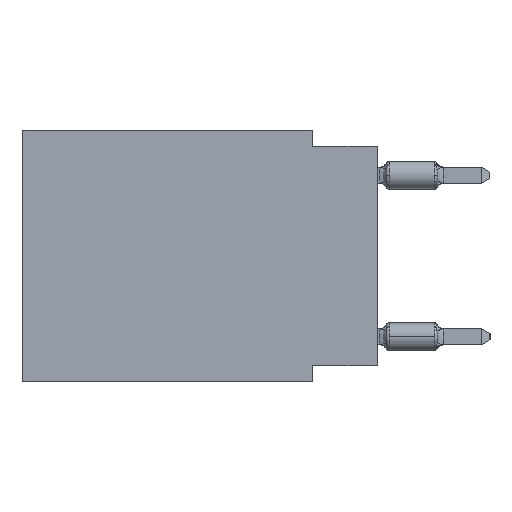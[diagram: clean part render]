
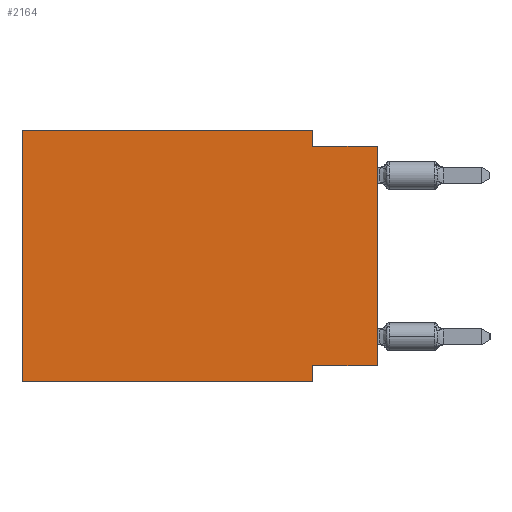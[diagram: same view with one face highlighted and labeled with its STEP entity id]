
A CAD part, left-side view. The second image highlights one B-rep face of the part: STEP entity #2164.
In plain terms, the highlighted planar face has unit normal (-1, 0, 0).
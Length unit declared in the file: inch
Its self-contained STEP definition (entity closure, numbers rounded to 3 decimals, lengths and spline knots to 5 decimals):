
#713 = CARTESIAN_POINT ( 'NONE',  ( 0., 0., 0. ) ) ;
#2164 = ADVANCED_FACE ( 'NONE', ( #4835 ), #30822, .F. ) ;
#2809 = CARTESIAN_POINT ( 'NONE',  ( 0., 0.55, 0. ) ) ;
#2903 = VERTEX_POINT ( 'NONE', #6981 ) ;
#3348 = EDGE_CURVE ( 'NONE', #12321, #16263, #21961, .T. ) ;
#3411 = CARTESIAN_POINT ( 'NONE',  ( 0., 0.1, -0.39 ) ) ;
#3478 = CARTESIAN_POINT ( 'NONE',  ( 0., 0.1, -0.365 ) ) ;
#3516 = VERTEX_POINT ( 'NONE', #37759 ) ;
#4691 = LINE ( 'NONE', #11243, #46310 ) ;
#4835 = FACE_OUTER_BOUND ( 'NONE', #22548, .T. ) ;
#5545 = VECTOR ( 'NONE', #43351, 39.37008 ) ;
#6262 = AXIS2_PLACEMENT_3D ( 'NONE', #34240, #31296, #8716 ) ;
#6981 = CARTESIAN_POINT ( 'NONE',  ( 0., 0., -0.365 ) ) ;
#7005 = CARTESIAN_POINT ( 'NONE',  ( 0., 0.55, -0.39 ) ) ;
#8716 = DIRECTION ( 'NONE',  ( 0., 0., -1. ) ) ;
#8881 = EDGE_CURVE ( 'NONE', #2903, #16263, #44655, .T. ) ;
#9873 = CARTESIAN_POINT ( 'NONE',  ( 0., 0.1, -0.39 ) ) ;
#10056 = ORIENTED_EDGE ( 'NONE', *, *, #18883, .F. ) ;
#10548 = CARTESIAN_POINT ( 'NONE',  ( 0., 0., -0.025 ) ) ;
#10950 = LINE ( 'NONE', #25783, #45664 ) ;
#11243 = CARTESIAN_POINT ( 'NONE',  ( 0., 0.55, 0. ) ) ;
#11287 = EDGE_CURVE ( 'NONE', #3516, #16032, #31505, .T. ) ;
#12321 = VERTEX_POINT ( 'NONE', #26258 ) ;
#12491 = CARTESIAN_POINT ( 'NONE',  ( 0., 0., -0.025 ) ) ;
#13269 = DIRECTION ( 'NONE',  ( 0., 0., 1. ) ) ;
#13389 = ORIENTED_EDGE ( 'NONE', *, *, #41497, .T. ) ;
#16032 = VERTEX_POINT ( 'NONE', #2809 ) ;
#16173 = CARTESIAN_POINT ( 'NONE',  ( 0., 0.1, 0. ) ) ;
#16263 = VERTEX_POINT ( 'NONE', #12491 ) ;
#17025 = VECTOR ( 'NONE', #32814, 39.37008 ) ;
#18883 = EDGE_CURVE ( 'NONE', #31305, #30698, #44447, .T. ) ;
#19387 = EDGE_CURVE ( 'NONE', #47445, #12321, #32511, .T. ) ;
#21961 = LINE ( 'NONE', #10548, #5545 ) ;
#22127 = DIRECTION ( 'NONE',  ( 0., 1., 0. ) ) ;
#22436 = EDGE_CURVE ( 'NONE', #16032, #47445, #4691, .T. ) ;
#22548 = EDGE_LOOP ( 'NONE', ( #25503, #32218, #28110, #30426, #34931, #13389, #10056, #30839 ) ) ;
#23762 = DIRECTION ( 'NONE',  ( 0., 0., 1. ) ) ;
#25210 = DIRECTION ( 'NONE',  ( 0., 0., -1. ) ) ;
#25503 = ORIENTED_EDGE ( 'NONE', *, *, #8881, .T. ) ;
#25783 = CARTESIAN_POINT ( 'NONE',  ( 0., 0., -0.365 ) ) ;
#26258 = CARTESIAN_POINT ( 'NONE',  ( 0., 0.1, -0.025 ) ) ;
#28110 = ORIENTED_EDGE ( 'NONE', *, *, #19387, .F. ) ;
#30206 = DIRECTION ( 'NONE',  ( 0., -1., 0. ) ) ;
#30426 = ORIENTED_EDGE ( 'NONE', *, *, #22436, .F. ) ;
#30698 = VERTEX_POINT ( 'NONE', #9873 ) ;
#30822 = PLANE ( 'NONE',  #6262 ) ;
#30839 = ORIENTED_EDGE ( 'NONE', *, *, #36082, .F. ) ;
#31296 = DIRECTION ( 'NONE',  ( 1., 0., 0. ) ) ;
#31305 = VERTEX_POINT ( 'NONE', #3478 ) ;
#31505 = LINE ( 'NONE', #39271, #31785 ) ;
#31785 = VECTOR ( 'NONE', #13269, 39.37008 ) ;
#32218 = ORIENTED_EDGE ( 'NONE', *, *, #3348, .F. ) ;
#32511 = LINE ( 'NONE', #39550, #44769 ) ;
#32814 = DIRECTION ( 'NONE',  ( 0., 0., -1. ) ) ;
#34240 = CARTESIAN_POINT ( 'NONE',  ( 0., 0.55, 0. ) ) ;
#34931 = ORIENTED_EDGE ( 'NONE', *, *, #11287, .F. ) ;
#36082 = EDGE_CURVE ( 'NONE', #2903, #31305, #10950, .T. ) ;
#37759 = CARTESIAN_POINT ( 'NONE',  ( 0., 0.55, -0.39 ) ) ;
#39271 = CARTESIAN_POINT ( 'NONE',  ( 0., 0.55, 0. ) ) ;
#39313 = VECTOR ( 'NONE', #23762, 39.37008 ) ;
#39550 = CARTESIAN_POINT ( 'NONE',  ( 0., 0.1, 0. ) ) ;
#40265 = LINE ( 'NONE', #7005, #45212 ) ;
#41497 = EDGE_CURVE ( 'NONE', #3516, #30698, #40265, .T. ) ;
#43351 = DIRECTION ( 'NONE',  ( 0., -1., 0. ) ) ;
#44447 = LINE ( 'NONE', #3411, #17025 ) ;
#44655 = LINE ( 'NONE', #713, #39313 ) ;
#44769 = VECTOR ( 'NONE', #25210, 39.37008 ) ;
#45212 = VECTOR ( 'NONE', #47482, 39.37008 ) ;
#45664 = VECTOR ( 'NONE', #22127, 39.37008 ) ;
#46310 = VECTOR ( 'NONE', #30206, 39.37008 ) ;
#47445 = VERTEX_POINT ( 'NONE', #16173 ) ;
#47482 = DIRECTION ( 'NONE',  ( 0., -1., 0. ) ) ;
